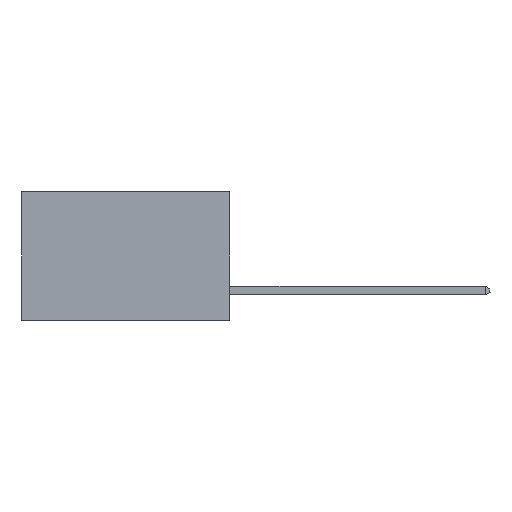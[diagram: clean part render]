
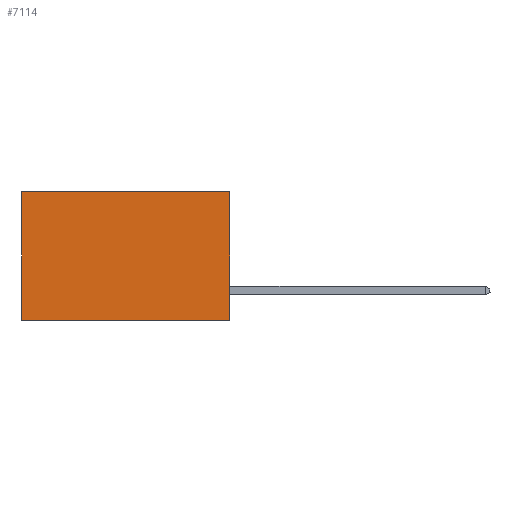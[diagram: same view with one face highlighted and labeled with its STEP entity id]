
A CAD part, left-side view. The second image highlights one B-rep face of the part: STEP entity #7114.
In plain terms, the highlighted planar face has unit normal (-1, 0, 0).
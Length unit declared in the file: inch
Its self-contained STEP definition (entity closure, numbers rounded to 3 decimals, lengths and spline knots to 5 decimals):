
#216 = CARTESIAN_POINT ( 'NONE',  ( 0.298, 0., -0.37 ) ) ;
#397 = LINE ( 'NONE', #2403, #9311 ) ;
#815 = VECTOR ( 'NONE', #960, 39.37008 ) ;
#960 = DIRECTION ( 'NONE',  ( 0., 0., -1. ) ) ;
#1520 = DIRECTION ( 'NONE',  ( 1., 0., 0. ) ) ;
#1638 = AXIS2_PLACEMENT_3D ( 'NONE', #9256, #1520, #2311 ) ;
#1773 = CARTESIAN_POINT ( 'NONE',  ( 0.298, 0., 0. ) ) ;
#1825 = ORIENTED_EDGE ( 'NONE', *, *, #3383, .T. ) ;
#2311 = DIRECTION ( 'NONE',  ( 0., 0., -1. ) ) ;
#2403 = CARTESIAN_POINT ( 'NONE',  ( 0.298, 0., -0.37 ) ) ;
#3383 = EDGE_CURVE ( 'NONE', #6529, #10076, #6948, .T. ) ;
#3404 = CARTESIAN_POINT ( 'NONE',  ( 0.298, 0., 0. ) ) ;
#3674 = DIRECTION ( 'NONE',  ( 0., 0., -1. ) ) ;
#3842 = ORIENTED_EDGE ( 'NONE', *, *, #5046, .T. ) ;
#4220 = LINE ( 'NONE', #1773, #815 ) ;
#4672 = VECTOR ( 'NONE', #9413, 39.37008 ) ;
#5046 = EDGE_CURVE ( 'NONE', #10076, #10420, #10369, .T. ) ;
#5618 = EDGE_CURVE ( 'NONE', #6529, #6850, #4220, .T. ) ;
#5837 = VECTOR ( 'NONE', #3674, 39.37008 ) ;
#5965 = CARTESIAN_POINT ( 'NONE',  ( 0.298, 0.6, 0. ) ) ;
#6529 = VERTEX_POINT ( 'NONE', #10551 ) ;
#6850 = VERTEX_POINT ( 'NONE', #216 ) ;
#6948 = LINE ( 'NONE', #3404, #4672 ) ;
#6977 = EDGE_CURVE ( 'NONE', #6850, #10420, #397, .T. ) ;
#7114 = ADVANCED_FACE ( 'NONE', ( #10598 ), #9798, .F. ) ;
#7439 = DIRECTION ( 'NONE',  ( 0., 1., 0. ) ) ;
#7769 = EDGE_LOOP ( 'NONE', ( #3842, #9371, #10897, #1825 ) ) ;
#8076 = CARTESIAN_POINT ( 'NONE',  ( 0.298, 0.6, -0.37 ) ) ;
#8810 = CARTESIAN_POINT ( 'NONE',  ( 0.298, 0.6, 0. ) ) ;
#9256 = CARTESIAN_POINT ( 'NONE',  ( 0.298, 0., 0. ) ) ;
#9311 = VECTOR ( 'NONE', #7439, 39.37008 ) ;
#9371 = ORIENTED_EDGE ( 'NONE', *, *, #6977, .F. ) ;
#9413 = DIRECTION ( 'NONE',  ( 0., 1., 0. ) ) ;
#9798 = PLANE ( 'NONE',  #1638 ) ;
#10076 = VERTEX_POINT ( 'NONE', #5965 ) ;
#10369 = LINE ( 'NONE', #8810, #5837 ) ;
#10420 = VERTEX_POINT ( 'NONE', #8076 ) ;
#10551 = CARTESIAN_POINT ( 'NONE',  ( 0.298, 0., 0. ) ) ;
#10598 = FACE_OUTER_BOUND ( 'NONE', #7769, .T. ) ;
#10897 = ORIENTED_EDGE ( 'NONE', *, *, #5618, .F. ) ;
